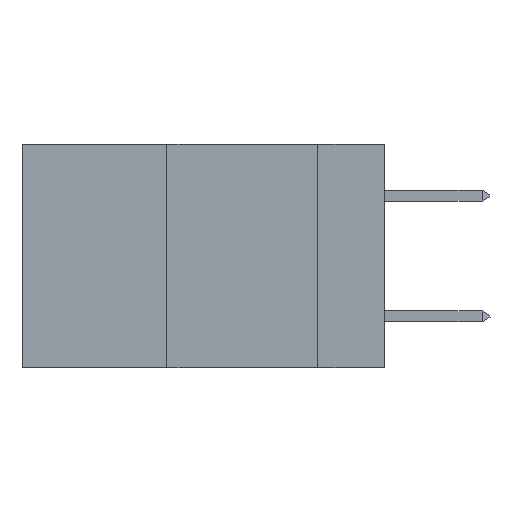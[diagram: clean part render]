
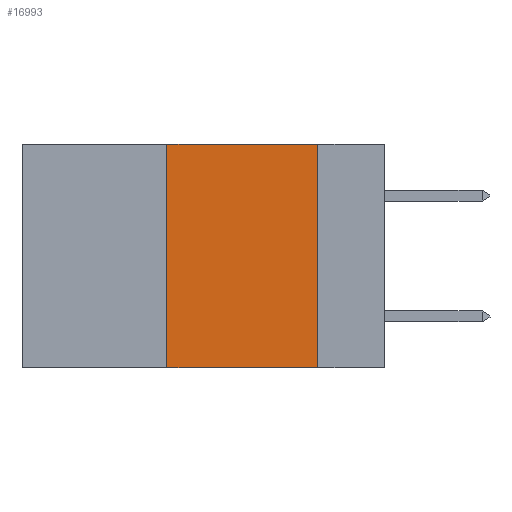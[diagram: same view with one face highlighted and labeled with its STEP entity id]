
A CAD part, left-side view. The second image highlights one B-rep face of the part: STEP entity #16993.
In plain terms, the highlighted planar face has unit normal (-1, 0, 0).
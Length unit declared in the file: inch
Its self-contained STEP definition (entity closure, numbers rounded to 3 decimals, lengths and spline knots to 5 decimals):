
#384 = LINE ( 'NONE', #14872, #23091 ) ;
#879 = VECTOR ( 'NONE', #18282, 39.37008 ) ;
#1578 = EDGE_CURVE ( 'NONE', #20227, #17411, #384, .T. ) ;
#3049 = DIRECTION ( 'NONE',  ( 0., 0., 1. ) ) ;
#3443 = CARTESIAN_POINT ( 'NONE',  ( 0., 0.6, 0. ) ) ;
#5306 = PLANE ( 'NONE',  #8391 ) ;
#6309 = LINE ( 'NONE', #9402, #879 ) ;
#6386 = LINE ( 'NONE', #7729, #10648 ) ;
#6555 = CARTESIAN_POINT ( 'NONE',  ( 0., 0.11, -0.37 ) ) ;
#7121 = DIRECTION ( 'NONE',  ( 0., 0., -1. ) ) ;
#7471 = CARTESIAN_POINT ( 'NONE',  ( 0., 0.11, 0. ) ) ;
#7729 = CARTESIAN_POINT ( 'NONE',  ( 0., 0.6, -0.37 ) ) ;
#8343 = EDGE_CURVE ( 'NONE', #16719, #20227, #6309, .T. ) ;
#8391 = AXIS2_PLACEMENT_3D ( 'NONE', #3443, #17835, #7121 ) ;
#8719 = ORIENTED_EDGE ( 'NONE', *, *, #17710, .T. ) ;
#9320 = VECTOR ( 'NONE', #3049, 39.37008 ) ;
#9402 = CARTESIAN_POINT ( 'NONE',  ( 0., 0.6, 0. ) ) ;
#10648 = VECTOR ( 'NONE', #18436, 39.37008 ) ;
#12410 = ORIENTED_EDGE ( 'NONE', *, *, #8343, .F. ) ;
#13136 = DIRECTION ( 'NONE',  ( 0., 0., -1. ) ) ;
#14230 = VERTEX_POINT ( 'NONE', #20952 ) ;
#14872 = CARTESIAN_POINT ( 'NONE',  ( 0., 0.11, 0. ) ) ;
#16719 = VERTEX_POINT ( 'NONE', #18871 ) ;
#16780 = FACE_OUTER_BOUND ( 'NONE', #20108, .T. ) ;
#16993 = ADVANCED_FACE ( 'NONE', ( #16780 ), #5306, .F. ) ;
#17411 = VERTEX_POINT ( 'NONE', #6555 ) ;
#17651 = ORIENTED_EDGE ( 'NONE', *, *, #21235, .F. ) ;
#17710 = EDGE_CURVE ( 'NONE', #14230, #17411, #6386, .T. ) ;
#17835 = DIRECTION ( 'NONE',  ( 1., 0., 0. ) ) ;
#18282 = DIRECTION ( 'NONE',  ( 0., -1., 0. ) ) ;
#18436 = DIRECTION ( 'NONE',  ( 0., -1., 0. ) ) ;
#18806 = LINE ( 'NONE', #19141, #9320 ) ;
#18871 = CARTESIAN_POINT ( 'NONE',  ( 0., 0.36, 0. ) ) ;
#19141 = CARTESIAN_POINT ( 'NONE',  ( 0., 0.36, 0. ) ) ;
#20108 = EDGE_LOOP ( 'NONE', ( #20684, #12410, #17651, #8719 ) ) ;
#20227 = VERTEX_POINT ( 'NONE', #7471 ) ;
#20684 = ORIENTED_EDGE ( 'NONE', *, *, #1578, .F. ) ;
#20952 = CARTESIAN_POINT ( 'NONE',  ( 0., 0.36, -0.37 ) ) ;
#21235 = EDGE_CURVE ( 'NONE', #14230, #16719, #18806, .T. ) ;
#23091 = VECTOR ( 'NONE', #13136, 39.37008 ) ;
